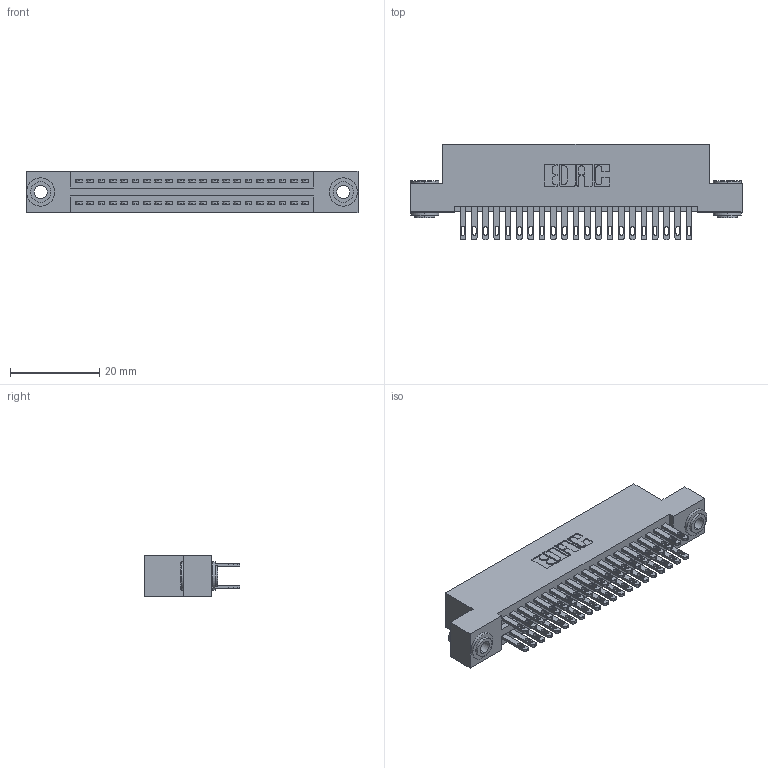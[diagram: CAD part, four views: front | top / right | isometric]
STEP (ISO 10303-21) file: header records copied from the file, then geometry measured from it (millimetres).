
FILE_DESCRIPTION (( 'STEP AP203' ), '1' );
FILE_NAME ('345-042-500-203.STEP', '2018-09-05T10:01:46', ( '' ), ( '' ), 'SwSTEP 2.0', 'SolidWorks 2016', '' );
FILE_SCHEMA (( 'CONFIG_CONTROL_DESIGN' ));
Length unit declared in the file: inch
Products named in the file (4): 345 Part_Flush Mounting Lugs - 0.156 Dia-TH; 345-292-001_345-293-100; 345-250-002_345-250-002-102; 345-042-500-203
Assembly tree (45 placements, depth 2):
  345-042-500-203
    345 Part_Flush Mounting Lugs - 0.156 Dia-TH
    345-292-001_345-293-100  x42
    345-250-002_345-250-002-102  x2
Bounding box: 74.55 x 21.51 x 9.4 mm (x, y, z)
Volume: 7194.6 mm3; surface area: 10861.3 mm2
Topology: 45 solids, 45 shells, 2096 faces, 6339 edges, 4222 vertices
Faces by surface type: plane 1224, cylinder 864, cone 8
Entity records: 19884 total; most frequent: CARTESIAN_POINT 3327, ORIENTED_EDGE 3254, DIRECTION 2993, EDGE_CURVE 1627, VECTOR 1383, LINE 1383, VERTEX_POINT 1082, AXIS2_PLACEMENT_3D 805
